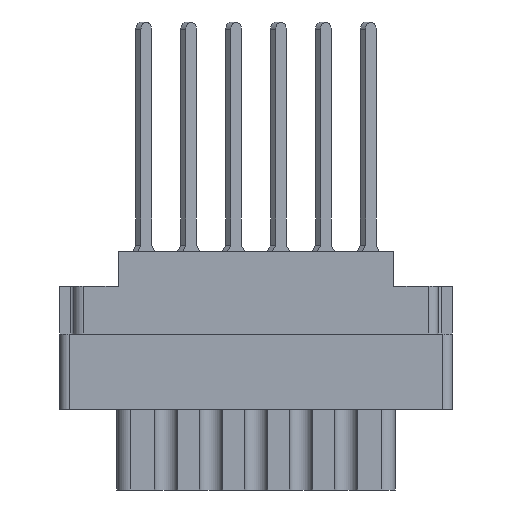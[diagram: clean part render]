
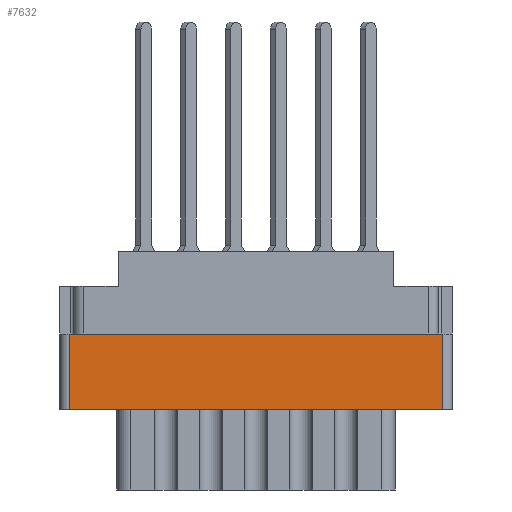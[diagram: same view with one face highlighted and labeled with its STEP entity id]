
A CAD part, front view. The second image highlights one B-rep face of the part: STEP entity #7632.
In plain terms, the highlighted planar face has unit normal (0, -1, 0).
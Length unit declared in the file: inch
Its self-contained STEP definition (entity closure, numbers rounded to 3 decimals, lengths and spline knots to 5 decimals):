
#250 = EDGE_CURVE ( 'NONE', #16874, #15269, #15084, .T. ) ;
#613 = CARTESIAN_POINT ( 'NONE',  ( -0.624, -0.343, -0.798 ) ) ;
#1165 = VERTEX_POINT ( 'NONE', #13971 ) ;
#1205 = EDGE_LOOP ( 'NONE', ( #2418, #4882, #17529, #5261 ) ) ;
#1701 = DIRECTION ( 'NONE',  ( -1., 0., 0. ) ) ;
#1945 = AXIS2_PLACEMENT_3D ( 'NONE', #12670, #15857, #3734 ) ;
#2155 = LINE ( 'NONE', #613, #5608 ) ;
#2418 = ORIENTED_EDGE ( 'NONE', *, *, #11266, .F. ) ;
#3032 = DIRECTION ( 'NONE',  ( 0., 0., 1. ) ) ;
#3734 = DIRECTION ( 'NONE',  ( 0., 0., -1. ) ) ;
#3758 = VECTOR ( 'NONE', #5930, 39.37008 ) ;
#4027 = FACE_OUTER_BOUND ( 'NONE', #1205, .T. ) ;
#4882 = ORIENTED_EDGE ( 'NONE', *, *, #250, .F. ) ;
#5261 = ORIENTED_EDGE ( 'NONE', *, *, #10995, .F. ) ;
#5608 = VECTOR ( 'NONE', #12540, 39.37008 ) ;
#5930 = DIRECTION ( 'NONE',  ( 1., 0., 0. ) ) ;
#5944 = VERTEX_POINT ( 'NONE', #11938 ) ;
#7632 = ADVANCED_FACE ( 'NONE', ( #4027 ), #8001, .T. ) ;
#8001 = PLANE ( 'NONE',  #1945 ) ;
#8373 = VECTOR ( 'NONE', #1701, 39.37008 ) ;
#10957 = EDGE_CURVE ( 'NONE', #16874, #5944, #17572, .T. ) ;
#10995 = EDGE_CURVE ( 'NONE', #1165, #5944, #11581, .T. ) ;
#11266 = EDGE_CURVE ( 'NONE', #15269, #1165, #2155, .T. ) ;
#11581 = LINE ( 'NONE', #17674, #3758 ) ;
#11938 = CARTESIAN_POINT ( 'NONE',  ( 0.624, -0.343, -0.277 ) ) ;
#12540 = DIRECTION ( 'NONE',  ( 0., 0., 1. ) ) ;
#12670 = CARTESIAN_POINT ( 'NONE',  ( -0.624, -0.343, -0.798 ) ) ;
#13032 = CARTESIAN_POINT ( 'NONE',  ( 0.624, -0.343, -0.798 ) ) ;
#13948 = CARTESIAN_POINT ( 'NONE',  ( 0.624, -0.343, -0.529 ) ) ;
#13971 = CARTESIAN_POINT ( 'NONE',  ( -0.624, -0.343, -0.277 ) ) ;
#13984 = VECTOR ( 'NONE', #3032, 39.37008 ) ;
#14994 = CARTESIAN_POINT ( 'NONE',  ( 0.624, -0.343, -0.529 ) ) ;
#15084 = LINE ( 'NONE', #14994, #8373 ) ;
#15269 = VERTEX_POINT ( 'NONE', #19154 ) ;
#15857 = DIRECTION ( 'NONE',  ( 0., -1., 0. ) ) ;
#16874 = VERTEX_POINT ( 'NONE', #13948 ) ;
#17529 = ORIENTED_EDGE ( 'NONE', *, *, #10957, .T. ) ;
#17572 = LINE ( 'NONE', #13032, #13984 ) ;
#17674 = CARTESIAN_POINT ( 'NONE',  ( -0.656, -0.343, -0.277 ) ) ;
#19154 = CARTESIAN_POINT ( 'NONE',  ( -0.624, -0.343, -0.529 ) ) ;
